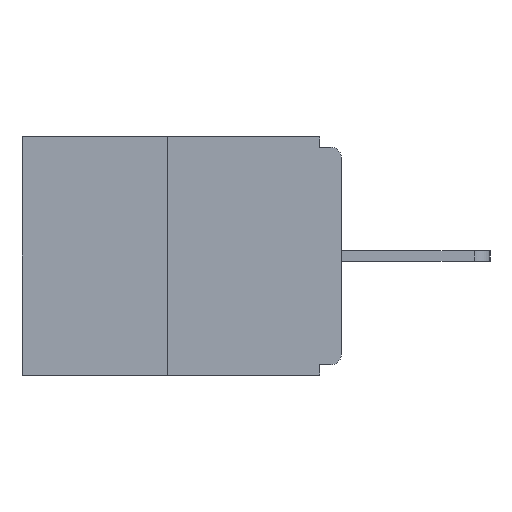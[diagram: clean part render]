
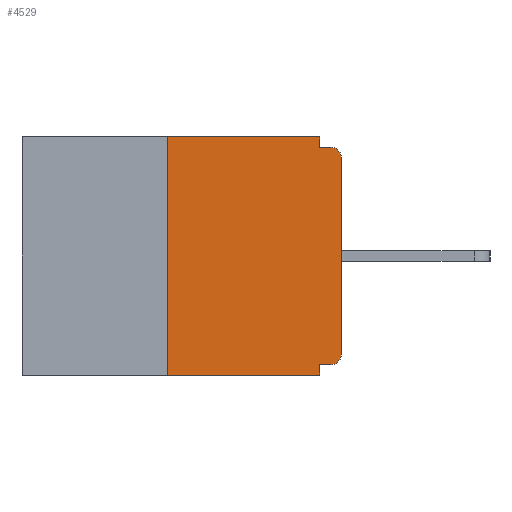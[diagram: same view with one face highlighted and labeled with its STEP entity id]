
A CAD part, left-side view. The second image highlights one B-rep face of the part: STEP entity #4529.
In plain terms, the highlighted planar face has unit normal (-1, 0, 0).
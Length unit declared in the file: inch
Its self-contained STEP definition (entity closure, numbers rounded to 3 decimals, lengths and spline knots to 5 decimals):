
#83 = CARTESIAN_POINT ( 'NONE',  ( 0., 0., 0. ) ) ;
#229 = ORIENTED_EDGE ( 'NONE', *, *, #3763, .T. ) ;
#372 = ORIENTED_EDGE ( 'NONE', *, *, #521, .F. ) ;
#491 = VERTEX_POINT ( 'NONE', #5535 ) ;
#521 = EDGE_CURVE ( 'NONE', #1821, #2308, #11787, .T. ) ;
#727 = DIRECTION ( 'NONE',  ( 0., 0., -1. ) ) ;
#749 = FACE_OUTER_BOUND ( 'NONE', #10120, .T. ) ;
#790 = CARTESIAN_POINT ( 'NONE',  ( 0., 0.031, 0. ) ) ;
#829 = LINE ( 'NONE', #15143, #1613 ) ;
#852 = CARTESIAN_POINT ( 'NONE',  ( 0., 0.46, 0. ) ) ;
#939 = DIRECTION ( 'NONE',  ( 0., -1., 0. ) ) ;
#1351 = EDGE_CURVE ( 'NONE', #3519, #1821, #2517, .T. ) ;
#1613 = VECTOR ( 'NONE', #2393, 39.37008 ) ;
#1821 = VERTEX_POINT ( 'NONE', #9717 ) ;
#1869 = EDGE_CURVE ( 'NONE', #13585, #9047, #7291, .T. ) ;
#1963 = CIRCLE ( 'NONE', #7748, 0.015 ) ;
#2161 = EDGE_CURVE ( 'NONE', #6433, #10897, #829, .T. ) ;
#2308 = VERTEX_POINT ( 'NONE', #3565 ) ;
#2393 = DIRECTION ( 'NONE',  ( 0., -1., 0. ) ) ;
#2431 = ORIENTED_EDGE ( 'NONE', *, *, #2832, .F. ) ;
#2517 = LINE ( 'NONE', #13089, #9195 ) ;
#2540 = EDGE_CURVE ( 'NONE', #491, #2308, #8014, .T. ) ;
#2832 = EDGE_CURVE ( 'NONE', #14342, #12406, #8066, .T. ) ;
#2852 = CARTESIAN_POINT ( 'NONE',  ( 0., 0., -0.313 ) ) ;
#2942 = PLANE ( 'NONE',  #4784 ) ;
#3482 = LINE ( 'NONE', #15452, #3952 ) ;
#3519 = VERTEX_POINT ( 'NONE', #3788 ) ;
#3565 = CARTESIAN_POINT ( 'NONE',  ( 0., 0.031, -0.343 ) ) ;
#3763 = EDGE_CURVE ( 'NONE', #9047, #10897, #1963, .T. ) ;
#3788 = CARTESIAN_POINT ( 'NONE',  ( 0., 0.015, -0.328 ) ) ;
#3888 = VECTOR ( 'NONE', #11807, 39.37008 ) ;
#3952 = VECTOR ( 'NONE', #9523, 39.37008 ) ;
#4386 = CARTESIAN_POINT ( 'NONE',  ( 0., 0.46, -0.343 ) ) ;
#4442 = CARTESIAN_POINT ( 'NONE',  ( 0., 0.015, -0.015 ) ) ;
#4529 = ADVANCED_FACE ( 'NONE', ( #749 ), #2942, .F. ) ;
#4784 = AXIS2_PLACEMENT_3D ( 'NONE', #5578, #13810, #7740 ) ;
#4860 = VECTOR ( 'NONE', #9449, 39.37008 ) ;
#5535 = CARTESIAN_POINT ( 'NONE',  ( 0., 0.25, -0.343 ) ) ;
#5542 = ORIENTED_EDGE ( 'NONE', *, *, #2540, .T. ) ;
#5578 = CARTESIAN_POINT ( 'NONE',  ( 0., 0.46, 0. ) ) ;
#5733 = CARTESIAN_POINT ( 'NONE',  ( 0., 0.031, -0.015 ) ) ;
#6191 = CARTESIAN_POINT ( 'NONE',  ( 0., 0.25, 0. ) ) ;
#6291 = DIRECTION ( 'NONE',  ( 0., 0., -1. ) ) ;
#6433 = VERTEX_POINT ( 'NONE', #5733 ) ;
#6878 = CARTESIAN_POINT ( 'NONE',  ( 0., 0., -0.03 ) ) ;
#7230 = CIRCLE ( 'NONE', #9216, 0.015 ) ;
#7291 = LINE ( 'NONE', #83, #3888 ) ;
#7298 = ORIENTED_EDGE ( 'NONE', *, *, #1351, .F. ) ;
#7740 = DIRECTION ( 'NONE',  ( 0., 0., -1. ) ) ;
#7748 = AXIS2_PLACEMENT_3D ( 'NONE', #14813, #8875, #727 ) ;
#8014 = LINE ( 'NONE', #4386, #8541 ) ;
#8066 = LINE ( 'NONE', #852, #10011 ) ;
#8541 = VECTOR ( 'NONE', #10513, 39.37008 ) ;
#8631 = CARTESIAN_POINT ( 'NONE',  ( 0., 0.015, -0.313 ) ) ;
#8875 = DIRECTION ( 'NONE',  ( -1., 0., 0. ) ) ;
#9047 = VERTEX_POINT ( 'NONE', #6878 ) ;
#9195 = VECTOR ( 'NONE', #13262, 39.37008 ) ;
#9216 = AXIS2_PLACEMENT_3D ( 'NONE', #8631, #13414, #6291 ) ;
#9449 = DIRECTION ( 'NONE',  ( 0., 0., -1. ) ) ;
#9523 = DIRECTION ( 'NONE',  ( 0., 0., 1. ) ) ;
#9708 = EDGE_CURVE ( 'NONE', #491, #14342, #3482, .T. ) ;
#9717 = CARTESIAN_POINT ( 'NONE',  ( 0., 0.031, -0.328 ) ) ;
#10011 = VECTOR ( 'NONE', #939, 39.37008 ) ;
#10120 = EDGE_LOOP ( 'NONE', ( #2431, #12838, #5542, #372, #7298, #13897, #11968, #229, #12486, #13257 ) ) ;
#10513 = DIRECTION ( 'NONE',  ( 0., -1., 0. ) ) ;
#10699 = CARTESIAN_POINT ( 'NONE',  ( 0., 0.031, -0.343 ) ) ;
#10897 = VERTEX_POINT ( 'NONE', #4442 ) ;
#11399 = EDGE_CURVE ( 'NONE', #3519, #13585, #7230, .T. ) ;
#11787 = LINE ( 'NONE', #10699, #13656 ) ;
#11807 = DIRECTION ( 'NONE',  ( 0., 0., 1. ) ) ;
#11859 = CARTESIAN_POINT ( 'NONE',  ( 0., 0.031, 0. ) ) ;
#11968 = ORIENTED_EDGE ( 'NONE', *, *, #1869, .T. ) ;
#12231 = EDGE_CURVE ( 'NONE', #12406, #6433, #13214, .T. ) ;
#12406 = VERTEX_POINT ( 'NONE', #790 ) ;
#12486 = ORIENTED_EDGE ( 'NONE', *, *, #2161, .F. ) ;
#12838 = ORIENTED_EDGE ( 'NONE', *, *, #9708, .F. ) ;
#13089 = CARTESIAN_POINT ( 'NONE',  ( 0., 0., -0.328 ) ) ;
#13214 = LINE ( 'NONE', #11859, #4860 ) ;
#13257 = ORIENTED_EDGE ( 'NONE', *, *, #12231, .F. ) ;
#13262 = DIRECTION ( 'NONE',  ( 0., 1., 0. ) ) ;
#13414 = DIRECTION ( 'NONE',  ( -1., 0., 0. ) ) ;
#13585 = VERTEX_POINT ( 'NONE', #2852 ) ;
#13656 = VECTOR ( 'NONE', #15460, 39.37008 ) ;
#13810 = DIRECTION ( 'NONE',  ( 1., 0., 0. ) ) ;
#13897 = ORIENTED_EDGE ( 'NONE', *, *, #11399, .T. ) ;
#14342 = VERTEX_POINT ( 'NONE', #6191 ) ;
#14813 = CARTESIAN_POINT ( 'NONE',  ( 0., 0.015, -0.03 ) ) ;
#15143 = CARTESIAN_POINT ( 'NONE',  ( 0., 0., -0.015 ) ) ;
#15452 = CARTESIAN_POINT ( 'NONE',  ( 0., 0.25, 0. ) ) ;
#15460 = DIRECTION ( 'NONE',  ( 0., 0., -1. ) ) ;
